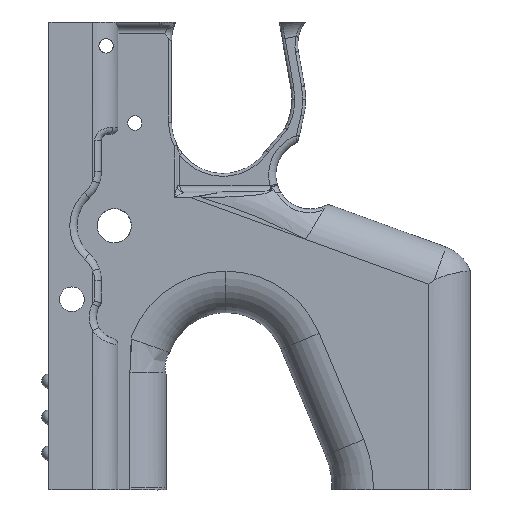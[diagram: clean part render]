
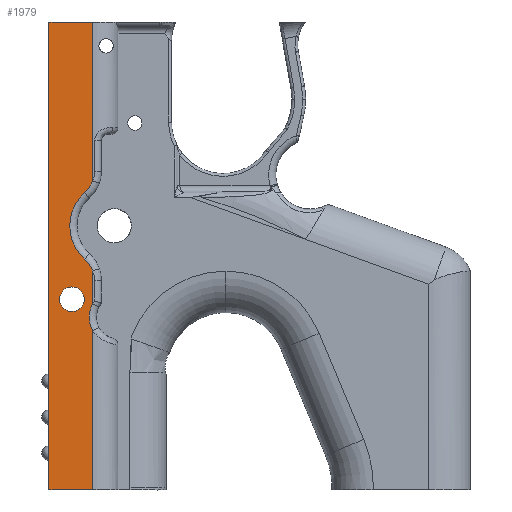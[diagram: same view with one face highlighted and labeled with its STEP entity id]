
A CAD part, left-side view. The second image highlights one B-rep face of the part: STEP entity #1979.
In plain terms, the highlighted planar face has unit normal (-1, 0, 0).
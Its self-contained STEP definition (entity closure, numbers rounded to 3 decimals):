
#35 = VERTEX_POINT ( 'NONE', #3280 ) ;
#245 = DIRECTION ( 'NONE',  ( 0., 0., 1. ) ) ;
#263 = PLANE ( 'NONE',  #3627 ) ;
#324 = VERTEX_POINT ( 'NONE', #12076 ) ;
#404 = CARTESIAN_POINT ( 'NONE',  ( -4.861, 21.06, 146.035 ) ) ;
#847 = VERTEX_POINT ( 'NONE', #7737 ) ;
#1063 = DIRECTION ( 'NONE',  ( -1., 0., 0. ) ) ;
#1094 = DIRECTION ( 'NONE',  ( 0., 0., 1. ) ) ;
#1127 = EDGE_CURVE ( 'NONE', #35, #6304, #12957, .T. ) ;
#1156 = LINE ( 'NONE', #3379, #9665 ) ;
#1325 = EDGE_LOOP ( 'NONE', ( #6548, #12789 ) ) ;
#1406 = FACE_OUTER_BOUND ( 'NONE', #2646, .T. ) ;
#1608 = VECTOR ( 'NONE', #7687, 1000. ) ;
#1711 = CARTESIAN_POINT ( 'NONE',  ( -4.861, 21.06, 82.636 ) ) ;
#1790 = DIRECTION ( 'NONE',  ( 0., 0., 1. ) ) ;
#1811 = LINE ( 'NONE', #6312, #2795 ) ;
#1979 = ADVANCED_FACE ( 'NONE', ( #6281, #1406 ), #263, .T. ) ;
#2265 = CARTESIAN_POINT ( 'NONE',  ( -4.861, 21.06, -3.178 ) ) ;
#2284 = CARTESIAN_POINT ( 'NONE',  ( -4.861, 21.06, 146.035 ) ) ;
#2305 = VECTOR ( 'NONE', #5846, 1000. ) ;
#2489 = EDGE_CURVE ( 'NONE', #13006, #8900, #10411, .T. ) ;
#2646 = EDGE_LOOP ( 'NONE', ( #5778, #9941, #11200, #9386, #4242, #3780, #11671, #8270, #3523, #4512 ) ) ;
#2742 = CARTESIAN_POINT ( 'NONE',  ( -4.861, 21.06, 4.399 ) ) ;
#2795 = VECTOR ( 'NONE', #12666, 1000. ) ;
#2818 = DIRECTION ( 'NONE',  ( 1., 0., 0. ) ) ;
#2913 = VERTEX_POINT ( 'NONE', #1711 ) ;
#3280 = CARTESIAN_POINT ( 'NONE',  ( -4.861, 26.817, 2.185 ) ) ;
#3354 = EDGE_CURVE ( 'NONE', #8900, #9213, #1156, .T. ) ;
#3379 = CARTESIAN_POINT ( 'NONE',  ( -4.861, 21.06, 146.035 ) ) ;
#3523 = ORIENTED_EDGE ( 'NONE', *, *, #3354, .T. ) ;
#3627 = AXIS2_PLACEMENT_3D ( 'NONE', #11150, #9012, #12170 ) ;
#3628 = DIRECTION ( 'NONE',  ( 1., 0., 0. ) ) ;
#3779 = CIRCLE ( 'NONE', #5392, 12.362 ) ;
#3780 = ORIENTED_EDGE ( 'NONE', *, *, #9969, .F. ) ;
#4019 = DIRECTION ( 'NONE',  ( 0., 0., 1. ) ) ;
#4242 = ORIENTED_EDGE ( 'NONE', *, *, #6187, .F. ) ;
#4393 = CARTESIAN_POINT ( 'NONE',  ( -4.861, 28.625, 41.182 ) ) ;
#4512 = ORIENTED_EDGE ( 'NONE', *, *, #12599, .T. ) ;
#4655 = CARTESIAN_POINT ( 'NONE',  ( -4.861, 21.06, 38.582 ) ) ;
#4929 = CARTESIAN_POINT ( 'NONE',  ( -4.861, 14.002, 0.611 ) ) ;
#4966 = AXIS2_PLACEMENT_3D ( 'NONE', #6123, #7647, #1094 ) ;
#4988 = CARTESIAN_POINT ( 'NONE',  ( -4.861, 28.625, 10.839 ) ) ;
#5260 = AXIS2_PLACEMENT_3D ( 'NONE', #4988, #12287, #6004 ) ;
#5308 = CARTESIAN_POINT ( 'NONE',  ( -4.861, 15.044, 26.011 ) ) ;
#5340 = CIRCLE ( 'NONE', #5863, 8. ) ;
#5392 = AXIS2_PLACEMENT_3D ( 'NONE', #5308, #2818, #10170 ) ;
#5500 = DIRECTION ( 'NONE',  ( 0., 0., 1. ) ) ;
#5548 = DIRECTION ( 'NONE',  ( 0., 0., 1. ) ) ;
#5549 = VECTOR ( 'NONE', #4019, 1000. ) ;
#5637 = CARTESIAN_POINT ( 'NONE',  ( -4.861, 26.817, 9.043 ) ) ;
#5653 = CIRCLE ( 'NONE', #5260, 8. ) ;
#5748 = EDGE_CURVE ( 'NONE', #6304, #35, #10339, .T. ) ;
#5778 = ORIENTED_EDGE ( 'NONE', *, *, #6018, .T. ) ;
#5846 = DIRECTION ( 'NONE',  ( 0., 1., 0. ) ) ;
#5863 = AXIS2_PLACEMENT_3D ( 'NONE', #4393, #1063, #5548 ) ;
#6004 = DIRECTION ( 'NONE',  ( 0., 0., 1. ) ) ;
#6018 = EDGE_CURVE ( 'NONE', #10407, #324, #3779, .T. ) ;
#6123 = CARTESIAN_POINT ( 'NONE',  ( -4.861, 26.817, 5.614 ) ) ;
#6187 = EDGE_CURVE ( 'NONE', #9848, #9715, #1811, .T. ) ;
#6281 = FACE_BOUND ( 'NONE', #1325, .T. ) ;
#6304 = VERTEX_POINT ( 'NONE', #5637 ) ;
#6312 = CARTESIAN_POINT ( 'NONE',  ( -4.861, 33.179, 167.539 ) ) ;
#6518 = EDGE_CURVE ( 'NONE', #2913, #9715, #10678, .T. ) ;
#6548 = ORIENTED_EDGE ( 'NONE', *, *, #5748, .F. ) ;
#6755 = EDGE_CURVE ( 'NONE', #847, #13006, #13202, .T. ) ;
#7256 = EDGE_CURVE ( 'NONE', #13492, #2913, #10047, .T. ) ;
#7319 = EDGE_CURVE ( 'NONE', #324, #13492, #5340, .T. ) ;
#7647 = DIRECTION ( 'NONE',  ( -1., 0., 0. ) ) ;
#7687 = DIRECTION ( 'NONE',  ( 0., 1., 0. ) ) ;
#7720 = DIRECTION ( 'NONE',  ( 0., 0., 1. ) ) ;
#7737 = CARTESIAN_POINT ( 'NONE',  ( -4.861, 21.06, -47.364 ) ) ;
#7960 = DIRECTION ( 'NONE',  ( -1., 0., 0. ) ) ;
#8270 = ORIENTED_EDGE ( 'NONE', *, *, #2489, .T. ) ;
#8650 = CARTESIAN_POINT ( 'NONE',  ( -4.861, 23.289, 16.8 ) ) ;
#8762 = CARTESIAN_POINT ( 'NONE',  ( -4.861, 21.06, 13.44 ) ) ;
#8900 = VERTEX_POINT ( 'NONE', #2742 ) ;
#8980 = AXIS2_PLACEMENT_3D ( 'NONE', #4929, #3628, #245 ) ;
#9012 = DIRECTION ( 'NONE',  ( -1., 0., 0. ) ) ;
#9213 = VERTEX_POINT ( 'NONE', #8762 ) ;
#9386 = ORIENTED_EDGE ( 'NONE', *, *, #6518, .T. ) ;
#9665 = VECTOR ( 'NONE', #5500, 1000. ) ;
#9715 = VERTEX_POINT ( 'NONE', #10496 ) ;
#9848 = VERTEX_POINT ( 'NONE', #13496 ) ;
#9941 = ORIENTED_EDGE ( 'NONE', *, *, #7319, .T. ) ;
#9969 = EDGE_CURVE ( 'NONE', #847, #9848, #13396, .T. ) ;
#10047 = LINE ( 'NONE', #404, #10159 ) ;
#10083 = CARTESIAN_POINT ( 'NONE',  ( -4.861, 26.817, 5.614 ) ) ;
#10159 = VECTOR ( 'NONE', #7720, 1000. ) ;
#10170 = DIRECTION ( 'NONE',  ( 0., 0., 1. ) ) ;
#10339 = CIRCLE ( 'NONE', #4966, 3.429 ) ;
#10407 = VERTEX_POINT ( 'NONE', #8650 ) ;
#10411 = CIRCLE ( 'NONE', #8980, 8.01 ) ;
#10496 = CARTESIAN_POINT ( 'NONE',  ( -4.861, 33.179, 82.636 ) ) ;
#10678 = LINE ( 'NONE', #12256, #2305 ) ;
#10801 = CARTESIAN_POINT ( 'NONE',  ( -4.861, 21.06, -47.364 ) ) ;
#11150 = CARTESIAN_POINT ( 'NONE',  ( -4.861, 21.06, 146.035 ) ) ;
#11200 = ORIENTED_EDGE ( 'NONE', *, *, #7256, .T. ) ;
#11671 = ORIENTED_EDGE ( 'NONE', *, *, #6755, .T. ) ;
#12076 = CARTESIAN_POINT ( 'NONE',  ( -4.861, 23.289, 35.222 ) ) ;
#12170 = DIRECTION ( 'NONE',  ( 0., 0., 1. ) ) ;
#12256 = CARTESIAN_POINT ( 'NONE',  ( -4.861, 21.06, 82.636 ) ) ;
#12287 = DIRECTION ( 'NONE',  ( -1., 0., 0. ) ) ;
#12599 = EDGE_CURVE ( 'NONE', #9213, #10407, #5653, .T. ) ;
#12666 = DIRECTION ( 'NONE',  ( 0., 0., 1. ) ) ;
#12789 = ORIENTED_EDGE ( 'NONE', *, *, #1127, .F. ) ;
#12957 = CIRCLE ( 'NONE', #13523, 3.429 ) ;
#13006 = VERTEX_POINT ( 'NONE', #2265 ) ;
#13202 = LINE ( 'NONE', #2284, #5549 ) ;
#13396 = LINE ( 'NONE', #10801, #1608 ) ;
#13492 = VERTEX_POINT ( 'NONE', #4655 ) ;
#13496 = CARTESIAN_POINT ( 'NONE',  ( -4.861, 33.179, -47.364 ) ) ;
#13523 = AXIS2_PLACEMENT_3D ( 'NONE', #10083, #7960, #1790 ) ;
